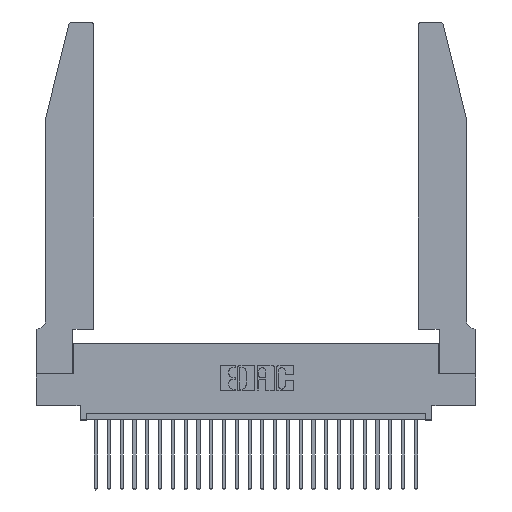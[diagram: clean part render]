
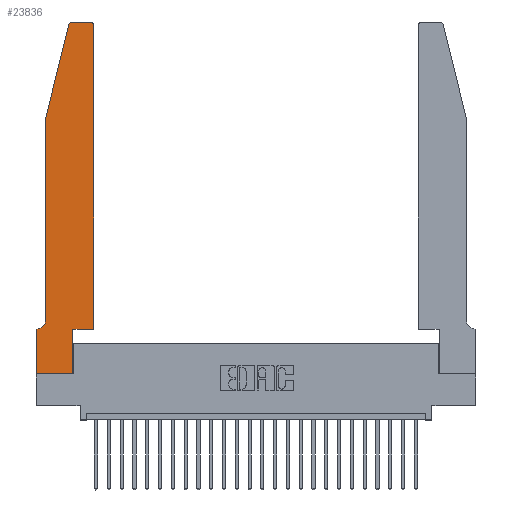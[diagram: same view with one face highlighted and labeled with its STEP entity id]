
A CAD part, top view. The second image highlights one B-rep face of the part: STEP entity #23836.
In plain terms, the highlighted planar face has unit normal (0, 0, 1).
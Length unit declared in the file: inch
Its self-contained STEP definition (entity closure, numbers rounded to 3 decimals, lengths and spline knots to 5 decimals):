
#300 = DIRECTION ( 'NONE',  ( 1., 0., 0. ) ) ;
#415 = DIRECTION ( 'NONE',  ( 1., 0., 0. ) ) ;
#464 = VERTEX_POINT ( 'NONE', #2842 ) ;
#564 = ORIENTED_EDGE ( 'NONE', *, *, #18975, .T. ) ;
#827 = EDGE_CURVE ( 'NONE', #11202, #20681, #26071, .T. ) ;
#836 = CARTESIAN_POINT ( 'NONE',  ( 0.0755, 0.42, 0.37 ) ) ;
#892 = ORIENTED_EDGE ( 'NONE', *, *, #827, .T. ) ;
#1066 = DIRECTION ( 'NONE',  ( 1., 0., 0. ) ) ;
#1231 = LINE ( 'NONE', #22865, #3477 ) ;
#1325 = CARTESIAN_POINT ( 'NONE',  ( 0., 0.35, 0.37 ) ) ;
#2295 = EDGE_CURVE ( 'NONE', #5893, #19007, #1231, .T. ) ;
#2499 = VERTEX_POINT ( 'NONE', #19704 ) ;
#2509 = AXIS2_PLACEMENT_3D ( 'NONE', #2895, #17208, #17121 ) ;
#2842 = CARTESIAN_POINT ( 'NONE',  ( 0.4205, 2.75, 0.37 ) ) ;
#2895 = CARTESIAN_POINT ( 'NONE',  ( 0.0055, 0.42, 0.37 ) ) ;
#3477 = VECTOR ( 'NONE', #415, 39.37008 ) ;
#3654 = DIRECTION ( 'NONE',  ( 1., 0., 0. ) ) ;
#3774 = FACE_OUTER_BOUND ( 'NONE', #8297, .T. ) ;
#3860 = EDGE_CURVE ( 'NONE', #464, #24299, #4673, .T. ) ;
#4125 = ORIENTED_EDGE ( 'NONE', *, *, #15646, .T. ) ;
#4673 = LINE ( 'NONE', #13658, #13299 ) ;
#5467 = DIRECTION ( 'NONE',  ( 0., 1., 0. ) ) ;
#5511 = PLANE ( 'NONE',  #19240 ) ;
#5861 = VERTEX_POINT ( 'NONE', #6742 ) ;
#5893 = VERTEX_POINT ( 'NONE', #22665 ) ;
#5916 = LINE ( 'NONE', #23963, #6240 ) ;
#6240 = VECTOR ( 'NONE', #5467, 39.37008 ) ;
#6601 = EDGE_CURVE ( 'NONE', #5861, #464, #6764, .T. ) ;
#6729 = VECTOR ( 'NONE', #10458, 39.37008 ) ;
#6742 = CARTESIAN_POINT ( 'NONE',  ( 0.4505, 2.72, 0.37 ) ) ;
#6764 = CIRCLE ( 'NONE', #19251, 0.03 ) ;
#6804 = ORIENTED_EDGE ( 'NONE', *, *, #18862, .T. ) ;
#7125 = ORIENTED_EDGE ( 'NONE', *, *, #21910, .T. ) ;
#7484 = LINE ( 'NONE', #20557, #11327 ) ;
#7739 = CIRCLE ( 'NONE', #14492, 0.03 ) ;
#8020 = ORIENTED_EDGE ( 'NONE', *, *, #2295, .T. ) ;
#8136 = CARTESIAN_POINT ( 'NONE',  ( 0., 0., 0.37 ) ) ;
#8248 = VERTEX_POINT ( 'NONE', #16203 ) ;
#8297 = EDGE_LOOP ( 'NONE', ( #24218, #19366, #24477, #7125, #892, #6804, #564, #25650, #4125, #8020, #10363, #13969 ) ) ;
#9823 = EDGE_CURVE ( 'NONE', #17741, #2499, #13111, .T. ) ;
#10142 = VECTOR ( 'NONE', #16313, 39.37008 ) ;
#10363 = ORIENTED_EDGE ( 'NONE', *, *, #23312, .T. ) ;
#10458 = DIRECTION ( 'NONE',  ( 0., -1., 0. ) ) ;
#10491 = CARTESIAN_POINT ( 'NONE',  ( 0.25487, 2.72718, 0.37 ) ) ;
#10536 = CARTESIAN_POINT ( 'NONE',  ( 0.4505, 0.35, 0.37 ) ) ;
#11158 = VECTOR ( 'NONE', #11408, 39.37008 ) ;
#11202 = VERTEX_POINT ( 'NONE', #836 ) ;
#11327 = VECTOR ( 'NONE', #16747, 39.37008 ) ;
#11408 = DIRECTION ( 'NONE',  ( 0., -1., 0. ) ) ;
#11722 = LINE ( 'NONE', #14582, #10142 ) ;
#13111 = LINE ( 'NONE', #15947, #14077 ) ;
#13299 = VECTOR ( 'NONE', #25862, 39.37008 ) ;
#13658 = CARTESIAN_POINT ( 'NONE',  ( 0.2605, 2.75, 0.37 ) ) ;
#13800 = CARTESIAN_POINT ( 'NONE',  ( 0.284, 2.72, 0.37 ) ) ;
#13969 = ORIENTED_EDGE ( 'NONE', *, *, #6601, .T. ) ;
#14077 = VECTOR ( 'NONE', #26529, 39.37008 ) ;
#14492 = AXIS2_PLACEMENT_3D ( 'NONE', #13800, #23827, #3654 ) ;
#14582 = CARTESIAN_POINT ( 'NONE',  ( 0.4505, 0.35, 0.37 ) ) ;
#15646 = EDGE_CURVE ( 'NONE', #2499, #5893, #5916, .T. ) ;
#15677 = LINE ( 'NONE', #19605, #11158 ) ;
#15824 = VERTEX_POINT ( 'NONE', #18007 ) ;
#15947 = CARTESIAN_POINT ( 'NONE',  ( 0., 0., 0.37 ) ) ;
#16203 = CARTESIAN_POINT ( 'NONE',  ( 0.0755, 2., 0.37 ) ) ;
#16313 = DIRECTION ( 'NONE',  ( 0., 1., 0. ) ) ;
#16321 = DIRECTION ( 'NONE',  ( -1., 0., 0. ) ) ;
#16747 = DIRECTION ( 'NONE',  ( -0.239, -0.971, 0. ) ) ;
#16881 = CARTESIAN_POINT ( 'NONE',  ( 0.0055, 0.35, 0.37 ) ) ;
#17121 = DIRECTION ( 'NONE',  ( -1., 0., 0. ) ) ;
#17208 = DIRECTION ( 'NONE',  ( 0., 0., -1. ) ) ;
#17741 = VERTEX_POINT ( 'NONE', #8136 ) ;
#18007 = CARTESIAN_POINT ( 'NONE',  ( 0., 0.35, 0.37 ) ) ;
#18010 = EDGE_CURVE ( 'NONE', #24299, #18406, #7739, .T. ) ;
#18390 = CARTESIAN_POINT ( 'NONE',  ( 0.0755, 0.35, 0.37 ) ) ;
#18406 = VERTEX_POINT ( 'NONE', #10491 ) ;
#18627 = VECTOR ( 'NONE', #16321, 39.37008 ) ;
#18862 = EDGE_CURVE ( 'NONE', #20681, #15824, #20884, .T. ) ;
#18877 = CARTESIAN_POINT ( 'NONE',  ( 0.284, 2.75, 0.37 ) ) ;
#18975 = EDGE_CURVE ( 'NONE', #15824, #17741, #20558, .T. ) ;
#19007 = VERTEX_POINT ( 'NONE', #10536 ) ;
#19240 = AXIS2_PLACEMENT_3D ( 'NONE', #1325, #23563, #1066 ) ;
#19251 = AXIS2_PLACEMENT_3D ( 'NONE', #22592, #24881, #300 ) ;
#19366 = ORIENTED_EDGE ( 'NONE', *, *, #18010, .T. ) ;
#19605 = CARTESIAN_POINT ( 'NONE',  ( 0.0755, 2., 0.37 ) ) ;
#19704 = CARTESIAN_POINT ( 'NONE',  ( 0.2865, 0., 0.37 ) ) ;
#20557 = CARTESIAN_POINT ( 'NONE',  ( 0.0755, 2., 0.37 ) ) ;
#20558 = LINE ( 'NONE', #21095, #6729 ) ;
#20681 = VERTEX_POINT ( 'NONE', #16881 ) ;
#20884 = LINE ( 'NONE', #18390, #18627 ) ;
#21095 = CARTESIAN_POINT ( 'NONE',  ( 0., 0., 0.37 ) ) ;
#21910 = EDGE_CURVE ( 'NONE', #8248, #11202, #15677, .T. ) ;
#22592 = CARTESIAN_POINT ( 'NONE',  ( 0.4205, 2.72, 0.37 ) ) ;
#22665 = CARTESIAN_POINT ( 'NONE',  ( 0.2865, 0.35, 0.37 ) ) ;
#22865 = CARTESIAN_POINT ( 'NONE',  ( 0.4505, 0.35, 0.37 ) ) ;
#23312 = EDGE_CURVE ( 'NONE', #19007, #5861, #11722, .T. ) ;
#23563 = DIRECTION ( 'NONE',  ( 0., 0., 1. ) ) ;
#23827 = DIRECTION ( 'NONE',  ( 0., 0., 1. ) ) ;
#23836 = ADVANCED_FACE ( 'NONE', ( #3774 ), #5511, .T. ) ;
#23963 = CARTESIAN_POINT ( 'NONE',  ( 0.2865, 0.35, 0.37 ) ) ;
#24218 = ORIENTED_EDGE ( 'NONE', *, *, #3860, .T. ) ;
#24299 = VERTEX_POINT ( 'NONE', #18877 ) ;
#24477 = ORIENTED_EDGE ( 'NONE', *, *, #25475, .T. ) ;
#24881 = DIRECTION ( 'NONE',  ( 0., 0., 1. ) ) ;
#25475 = EDGE_CURVE ( 'NONE', #18406, #8248, #7484, .T. ) ;
#25650 = ORIENTED_EDGE ( 'NONE', *, *, #9823, .T. ) ;
#25862 = DIRECTION ( 'NONE',  ( -1., 0., 0. ) ) ;
#26071 = CIRCLE ( 'NONE', #2509, 0.07 ) ;
#26529 = DIRECTION ( 'NONE',  ( 1., 0., 0. ) ) ;
